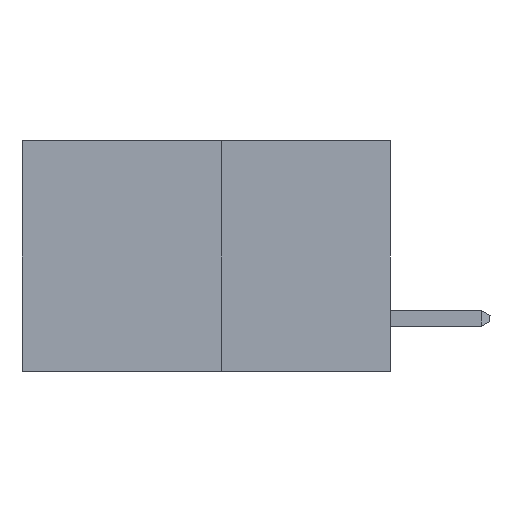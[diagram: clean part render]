
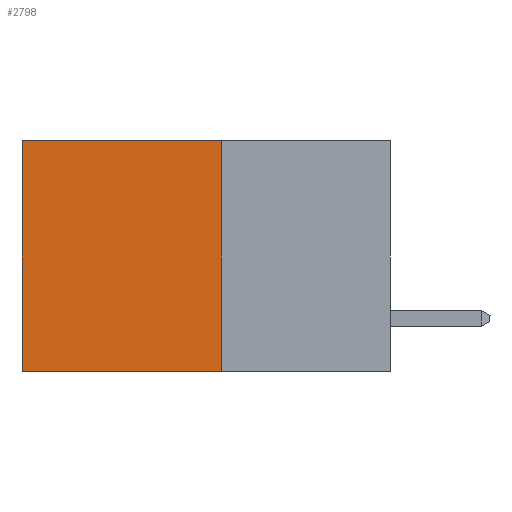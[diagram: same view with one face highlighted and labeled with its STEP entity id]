
A CAD part, left-side view. The second image highlights one B-rep face of the part: STEP entity #2798.
In plain terms, the highlighted planar face has unit normal (-1, 0, 0).
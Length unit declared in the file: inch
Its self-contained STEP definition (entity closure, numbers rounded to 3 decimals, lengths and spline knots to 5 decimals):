
#382 = EDGE_CURVE ( 'NONE', #15881, #10307, #8721, .T. ) ;
#2205 = ORIENTED_EDGE ( 'NONE', *, *, #6597, .T. ) ;
#2411 = CARTESIAN_POINT ( 'NONE',  ( 0.277, 0.27, -0.37 ) ) ;
#2798 = ADVANCED_FACE ( 'NONE', ( #22016 ), #12623, .F. ) ;
#3633 = DIRECTION ( 'NONE',  ( 0., 0., -1. ) ) ;
#4188 = CARTESIAN_POINT ( 'NONE',  ( 0.277, 0.27, 0. ) ) ;
#6597 = EDGE_CURVE ( 'NONE', #12090, #10307, #19262, .T. ) ;
#8525 = CARTESIAN_POINT ( 'NONE',  ( 0.277, 0.59, 0. ) ) ;
#8721 = LINE ( 'NONE', #17479, #13677 ) ;
#9214 = VECTOR ( 'NONE', #3633, 39.37008 ) ;
#10307 = VERTEX_POINT ( 'NONE', #24467 ) ;
#10537 = DIRECTION ( 'NONE',  ( 0., 1., 0. ) ) ;
#11366 = EDGE_CURVE ( 'NONE', #21223, #12090, #16300, .T. ) ;
#12090 = VERTEX_POINT ( 'NONE', #8525 ) ;
#12535 = DIRECTION ( 'NONE',  ( 1., 0., 0. ) ) ;
#12618 = CARTESIAN_POINT ( 'NONE',  ( 0.277, 0.27, -0.37 ) ) ;
#12623 = PLANE ( 'NONE',  #20047 ) ;
#13677 = VECTOR ( 'NONE', #17567, 39.37008 ) ;
#13710 = VECTOR ( 'NONE', #22535, 39.37008 ) ;
#15881 = VERTEX_POINT ( 'NONE', #2411 ) ;
#16300 = LINE ( 'NONE', #4188, #25959 ) ;
#16933 = CARTESIAN_POINT ( 'NONE',  ( 0.277, 0.27, 0. ) ) ;
#17023 = DIRECTION ( 'NONE',  ( 0., 0., -1. ) ) ;
#17479 = CARTESIAN_POINT ( 'NONE',  ( 0.277, 0.27, -0.37 ) ) ;
#17567 = DIRECTION ( 'NONE',  ( 0., 1., 0. ) ) ;
#17697 = EDGE_LOOP ( 'NONE', ( #2205, #26957, #23904, #26140 ) ) ;
#18406 = LINE ( 'NONE', #22568, #9214 ) ;
#19262 = LINE ( 'NONE', #22737, #13710 ) ;
#20047 = AXIS2_PLACEMENT_3D ( 'NONE', #12618, #12535, #17023 ) ;
#21223 = VERTEX_POINT ( 'NONE', #16933 ) ;
#22016 = FACE_OUTER_BOUND ( 'NONE', #17697, .T. ) ;
#22535 = DIRECTION ( 'NONE',  ( 0., 0., -1. ) ) ;
#22568 = CARTESIAN_POINT ( 'NONE',  ( 0.277, 0.27, -0.37 ) ) ;
#22737 = CARTESIAN_POINT ( 'NONE',  ( 0.277, 0.59, -0.37 ) ) ;
#22858 = EDGE_CURVE ( 'NONE', #21223, #15881, #18406, .T. ) ;
#23904 = ORIENTED_EDGE ( 'NONE', *, *, #22858, .F. ) ;
#24467 = CARTESIAN_POINT ( 'NONE',  ( 0.277, 0.59, -0.37 ) ) ;
#25959 = VECTOR ( 'NONE', #10537, 39.37008 ) ;
#26140 = ORIENTED_EDGE ( 'NONE', *, *, #11366, .T. ) ;
#26957 = ORIENTED_EDGE ( 'NONE', *, *, #382, .F. ) ;
